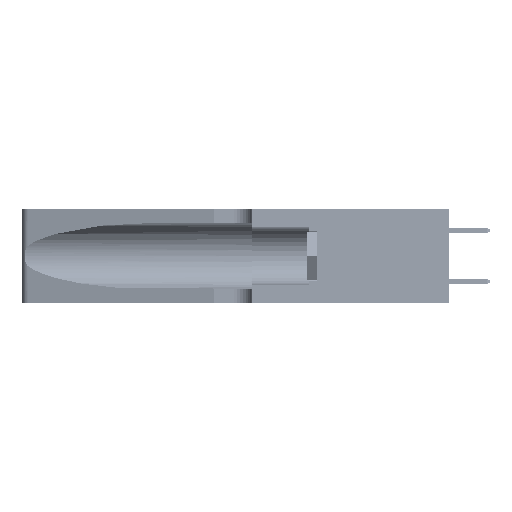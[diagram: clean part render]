
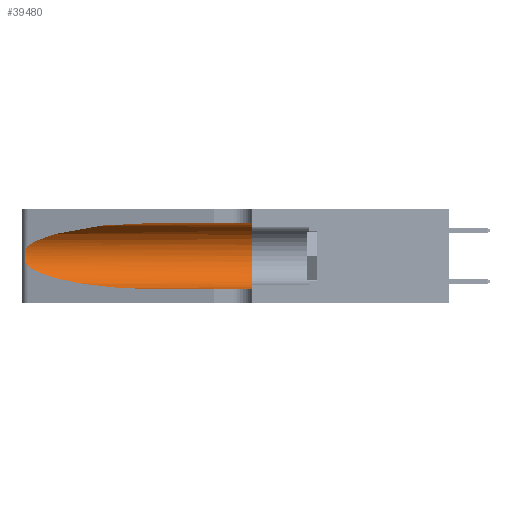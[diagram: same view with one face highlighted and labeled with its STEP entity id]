
A CAD part, left-side view. The second image highlights one B-rep face of the part: STEP entity #39480.
In plain terms, the highlighted cylindrical face has radius 3.308 mm (diameter 6.617 mm), a partial arc.
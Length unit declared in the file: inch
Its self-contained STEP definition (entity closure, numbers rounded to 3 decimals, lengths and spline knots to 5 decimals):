
#503 = VECTOR ( 'NONE', #47766, 39.37008 ) ;
#1002 = CARTESIAN_POINT ( 'NONE',  ( 0.1305, 0.72297, 0.05475 ) ) ;
#1416 = DIRECTION ( 'NONE',  ( 0., -1., 0. ) ) ;
#2235 = CARTESIAN_POINT ( 'NONE',  ( 0.1305, 0.72297, 0.31525 ) ) ;
#4182 = CARTESIAN_POINT ( 'NONE',  ( 0.25487, 1.22718, 0.22369 ) ) ;
#5304 = ORIENTED_EDGE ( 'NONE', *, *, #26425, .T. ) ;
#5562 = CARTESIAN_POINT ( 'NONE',  ( 0.1305, 0.35, 0.31525 ) ) ;
#6447 = CARTESIAN_POINT ( 'NONE',  ( 0.25787, 1.23484, 0.2124 ) ) ;
#7882 = EDGE_LOOP ( 'NONE', ( #29488, #5304, #10173, #15593, #28859, #33777 ) ) ;
#10173 = ORIENTED_EDGE ( 'NONE', *, *, #24939, .T. ) ;
#10543 = CARTESIAN_POINT ( 'NONE',  ( 0.26018, 1.23835, 0.19895 ) ) ;
#11854 = EDGE_CURVE ( 'NONE', #30774, #43760, #44807, .T. ) ;
#11920 = EDGE_CURVE ( 'NONE', #29576, #22637, #42581, .T. ) ;
#11951 = CYLINDRICAL_SURFACE ( 'NONE', #52400, 0.13025 ) ;
#13607 = DIRECTION ( 'NONE',  ( 0., 1., 0. ) ) ;
#14389 = CARTESIAN_POINT ( 'NONE',  ( 0.1305, 0.35, 0.05475 ) ) ;
#14722 = CARTESIAN_POINT ( 'NONE',  ( 0.26075, 1.23896, 0.178 ) ) ;
#15593 = ORIENTED_EDGE ( 'NONE', *, *, #48717, .T. ) ;
#17176 = VERTEX_POINT ( 'NONE', #21293 ) ;
#17879 = CARTESIAN_POINT ( 'NONE',  ( 0.18966, 0.96281, 0.31525 ) ) ;
#18814 = CARTESIAN_POINT ( 'NONE',  ( 0.25856, 1.23593, 0.16098 ) ) ;
#21293 = CARTESIAN_POINT ( 'NONE',  ( 0.25487, 1.22718, 0.14631 ) ) ;
#22043 = CARTESIAN_POINT ( 'NONE',  ( 0.25487, 1.22718, 0.22369 ) ) ;
#22373 = LINE ( 'NONE', #23394, #503 ) ;
#22637 = VERTEX_POINT ( 'NONE', #4182 ) ;
#22952 = CARTESIAN_POINT ( 'NONE',  ( 0.25639, 1.23186, 0.15144 ) ) ;
#23394 = CARTESIAN_POINT ( 'NONE',  ( 0.1305, 1.61858, 0.31525 ) ) ;
#23636 =( BOUNDED_CURVE ( )  B_SPLINE_CURVE ( 3, ( #33626, #41811, #25612, #1002 ),
 .UNSPECIFIED., .F., .F. ) 
 B_SPLINE_CURVE_WITH_KNOTS ( ( 4, 4 ),
 ( 3.44316, 4.71239 ),
 .UNSPECIFIED. ) 
 CURVE ( )  GEOMETRIC_REPRESENTATION_ITEM ( )  RATIONAL_B_SPLINE_CURVE ( ( 1., 0.87, 0.87, 1. ) ) 
 REPRESENTATION_ITEM ( '' )  );
#24939 = EDGE_CURVE ( 'NONE', #17176, #40534, #23636, .T. ) ;
#25612 = CARTESIAN_POINT ( 'NONE',  ( 0.18966, 0.96281, 0.05475 ) ) ;
#26022 = DIRECTION ( 'NONE',  ( 0., 0., -1. ) ) ;
#26425 = EDGE_CURVE ( 'NONE', #22637, #17176, #32829, .T. ) ;
#26698 = CARTESIAN_POINT ( 'NONE',  ( 0.1305, 0.72297, 0.05475 ) ) ;
#26755 = FACE_OUTER_BOUND ( 'NONE', #7882, .T. ) ;
#26911 = CARTESIAN_POINT ( 'NONE',  ( 0.25487, 1.22718, 0.22369 ) ) ;
#27092 = CARTESIAN_POINT ( 'NONE',  ( 0.25487, 1.22718, 0.14631 ) ) ;
#28859 = ORIENTED_EDGE ( 'NONE', *, *, #11854, .F. ) ;
#29488 = ORIENTED_EDGE ( 'NONE', *, *, #11920, .T. ) ;
#29576 = VERTEX_POINT ( 'NONE', #2235 ) ;
#30774 = VERTEX_POINT ( 'NONE', #5562 ) ;
#31018 = CARTESIAN_POINT ( 'NONE',  ( 0.25639, 1.23184, 0.21858 ) ) ;
#32829 = B_SPLINE_CURVE_WITH_KNOTS ( 'NONE', 3,
 ( #26911, #39026, #31018, #6447, #35108, #10543, #39199, #14722, #43265, #18814, #47350, #22952, #51407, #27092 ),
 .UNSPECIFIED., .F., .F.,
 ( 4, 2, 2, 2, 2, 2, 4 ),
 ( 0., 0.00027, 0.00053, 0.00107, 0.0016, 0.00187, 0.00214 ),
 .UNSPECIFIED. ) ;
#33626 = CARTESIAN_POINT ( 'NONE',  ( 0.25487, 1.22718, 0.14631 ) ) ;
#33777 = ORIENTED_EDGE ( 'NONE', *, *, #50164, .F. ) ;
#35108 = CARTESIAN_POINT ( 'NONE',  ( 0.25854, 1.2359, 0.20912 ) ) ;
#38093 = CARTESIAN_POINT ( 'NONE',  ( 0.1305, 0.35, 0.185 ) ) ;
#38262 = CARTESIAN_POINT ( 'NONE',  ( 0.2373, 1.15595, 0.28018 ) ) ;
#39026 = CARTESIAN_POINT ( 'NONE',  ( 0.25555, 1.22994, 0.2215 ) ) ;
#39199 = CARTESIAN_POINT ( 'NONE',  ( 0.26075, 1.23896, 0.19203 ) ) ;
#39480 = ADVANCED_FACE ( 'NONE', ( #26755 ), #11951, .F. ) ;
#40349 = VECTOR ( 'NONE', #44731, 39.37008 ) ;
#40534 = VERTEX_POINT ( 'NONE', #26698 ) ;
#40685 = CARTESIAN_POINT ( 'NONE',  ( 0.1305, 1.61858, 0.05475 ) ) ;
#41586 = LINE ( 'NONE', #40685, #40349 ) ;
#41811 = CARTESIAN_POINT ( 'NONE',  ( 0.2373, 1.15595, 0.08982 ) ) ;
#42168 = DIRECTION ( 'NONE',  ( 0., 0., 1. ) ) ;
#42581 =( BOUNDED_CURVE ( )  B_SPLINE_CURVE ( 3, ( #46426, #17879, #38262, #22043 ),
 .UNSPECIFIED., .F., .T. ) 
 B_SPLINE_CURVE_WITH_KNOTS ( ( 4, 4 ),
 ( 1.5708, 2.84003 ),
 .UNSPECIFIED. ) 
 CURVE ( )  GEOMETRIC_REPRESENTATION_ITEM ( )  RATIONAL_B_SPLINE_CURVE ( ( 1., 0.87, 0.87, 1. ) ) 
 REPRESENTATION_ITEM ( '' )  );
#43265 = CARTESIAN_POINT ( 'NONE',  ( 0.26017, 1.23833, 0.17102 ) ) ;
#43760 = VERTEX_POINT ( 'NONE', #14389 ) ;
#44731 = DIRECTION ( 'NONE',  ( 0., -1., 0. ) ) ;
#44807 = CIRCLE ( 'NONE', #51191, 0.13025 ) ;
#46426 = CARTESIAN_POINT ( 'NONE',  ( 0.1305, 0.72297, 0.31525 ) ) ;
#47350 = CARTESIAN_POINT ( 'NONE',  ( 0.25789, 1.23486, 0.15765 ) ) ;
#47766 = DIRECTION ( 'NONE',  ( 0., -1., 0. ) ) ;
#48717 = EDGE_CURVE ( 'NONE', #40534, #43760, #41586, .T. ) ;
#50164 = EDGE_CURVE ( 'NONE', #29576, #30774, #22373, .T. ) ;
#50342 = CARTESIAN_POINT ( 'NONE',  ( 0.1305, 1.61858, 0.185 ) ) ;
#51191 = AXIS2_PLACEMENT_3D ( 'NONE', #38093, #13607, #42168 ) ;
#51407 = CARTESIAN_POINT ( 'NONE',  ( 0.25555, 1.22993, 0.14849 ) ) ;
#52400 = AXIS2_PLACEMENT_3D ( 'NONE', #50342, #1416, #26022 ) ;
